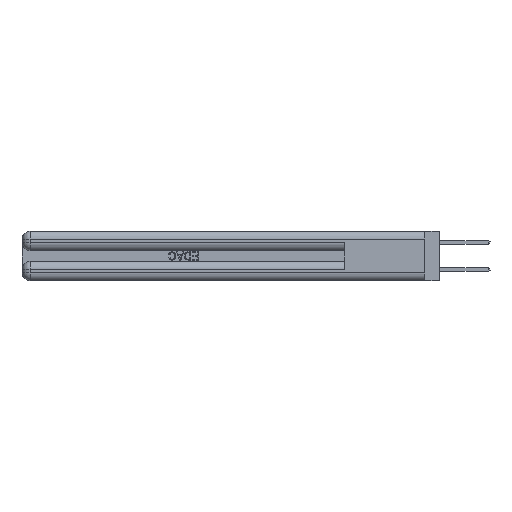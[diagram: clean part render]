
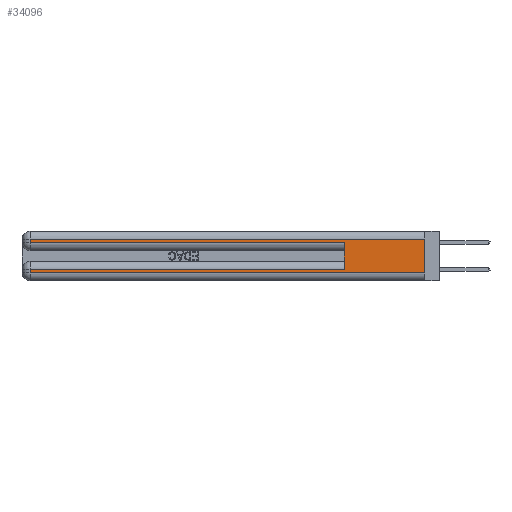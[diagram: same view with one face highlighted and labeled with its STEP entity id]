
A CAD part, left-side view. The second image highlights one B-rep face of the part: STEP entity #34096.
In plain terms, the highlighted planar face has unit normal (-1, 0, 0).
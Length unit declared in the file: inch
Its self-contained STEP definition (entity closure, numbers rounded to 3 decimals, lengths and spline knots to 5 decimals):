
#402 = ORIENTED_EDGE ( 'NONE', *, *, #39180, .T. ) ;
#793 = VERTEX_POINT ( 'NONE', #20027 ) ;
#1007 = EDGE_CURVE ( 'NONE', #11120, #20701, #22849, .T. ) ;
#1410 = LINE ( 'NONE', #12347, #18980 ) ;
#1851 = DIRECTION ( 'NONE',  ( 0., -1., 0. ) ) ;
#2838 = LINE ( 'NONE', #35011, #39089 ) ;
#2894 = ORIENTED_EDGE ( 'NONE', *, *, #20124, .T. ) ;
#4474 = CARTESIAN_POINT ( 'NONE',  ( 0., 2.94, 0.285 ) ) ;
#4774 = EDGE_CURVE ( 'NONE', #20701, #21897, #1410, .T. ) ;
#4783 = ORIENTED_EDGE ( 'NONE', *, *, #1007, .T. ) ;
#5353 = CARTESIAN_POINT ( 'NONE',  ( 0., 0.6, 0.145 ) ) ;
#5579 = CARTESIAN_POINT ( 'NONE',  ( 0., 2.94, 0.37 ) ) ;
#5633 = VERTEX_POINT ( 'NONE', #28132 ) ;
#5831 = CARTESIAN_POINT ( 'NONE',  ( 0., 0.6, 0.285 ) ) ;
#7106 = ORIENTED_EDGE ( 'NONE', *, *, #4774, .T. ) ;
#7929 = DIRECTION ( 'NONE',  ( 1., 0., 0. ) ) ;
#8664 = DIRECTION ( 'NONE',  ( 0., 0., -1. ) ) ;
#9414 = VERTEX_POINT ( 'NONE', #5831 ) ;
#10093 = VERTEX_POINT ( 'NONE', #29046 ) ;
#10469 = LINE ( 'NONE', #5353, #12691 ) ;
#11120 = VERTEX_POINT ( 'NONE', #17565 ) ;
#12266 = DIRECTION ( 'NONE',  ( 0., 1., 0. ) ) ;
#12347 = CARTESIAN_POINT ( 'NONE',  ( 0., 2.94, 0.37 ) ) ;
#12691 = VECTOR ( 'NONE', #19788, 39.37008 ) ;
#13507 = VECTOR ( 'NONE', #12266, 39.37008 ) ;
#14107 = EDGE_CURVE ( 'NONE', #10093, #793, #14462, .T. ) ;
#14462 = LINE ( 'NONE', #36508, #32043 ) ;
#17565 = CARTESIAN_POINT ( 'NONE',  ( 0., 0.6, 0.085 ) ) ;
#18980 = VECTOR ( 'NONE', #8664, 39.37008 ) ;
#19788 = DIRECTION ( 'NONE',  ( 0., 0., 1. ) ) ;
#19977 = EDGE_CURVE ( 'NONE', #793, #39813, #20931, .T. ) ;
#20027 = CARTESIAN_POINT ( 'NONE',  ( 0., 2.94, 0.31 ) ) ;
#20124 = EDGE_CURVE ( 'NONE', #21897, #5633, #37459, .T. ) ;
#20701 = VERTEX_POINT ( 'NONE', #36445 ) ;
#20931 = LINE ( 'NONE', #5579, #44081 ) ;
#21469 = PLANE ( 'NONE',  #40001 ) ;
#21581 = CARTESIAN_POINT ( 'NONE',  ( 0., 0., 0.285 ) ) ;
#21897 = VERTEX_POINT ( 'NONE', #40116 ) ;
#22849 = LINE ( 'NONE', #29802, #13507 ) ;
#23555 = DIRECTION ( 'NONE',  ( 0., 0., -1. ) ) ;
#23606 = ORIENTED_EDGE ( 'NONE', *, *, #19977, .T. ) ;
#25452 = DIRECTION ( 'NONE',  ( 0., 0., -1. ) ) ;
#28089 = DIRECTION ( 'NONE',  ( 0., 0., -1. ) ) ;
#28132 = CARTESIAN_POINT ( 'NONE',  ( 0., 0., 0.06 ) ) ;
#29046 = CARTESIAN_POINT ( 'NONE',  ( 0., 0., 0.31 ) ) ;
#29332 = FACE_OUTER_BOUND ( 'NONE', #40076, .T. ) ;
#29719 = EDGE_CURVE ( 'NONE', #10093, #5633, #2838, .T. ) ;
#29745 = DIRECTION ( 'NONE',  ( 0., -1., 0. ) ) ;
#29802 = CARTESIAN_POINT ( 'NONE',  ( 0., 0., 0.085 ) ) ;
#32043 = VECTOR ( 'NONE', #40526, 39.37008 ) ;
#34096 = ADVANCED_FACE ( 'NONE', ( #29332 ), #21469, .F. ) ;
#35011 = CARTESIAN_POINT ( 'NONE',  ( 0., 0., 0.37 ) ) ;
#36310 = VECTOR ( 'NONE', #1851, 39.37008 ) ;
#36445 = CARTESIAN_POINT ( 'NONE',  ( 0., 2.94, 0.085 ) ) ;
#36508 = CARTESIAN_POINT ( 'NONE',  ( 0., 0., 0.31 ) ) ;
#37459 = LINE ( 'NONE', #43812, #36310 ) ;
#38442 = ORIENTED_EDGE ( 'NONE', *, *, #44575, .F. ) ;
#39089 = VECTOR ( 'NONE', #28089, 39.37008 ) ;
#39156 = CARTESIAN_POINT ( 'NONE',  ( 0., 0., 0.37 ) ) ;
#39180 = EDGE_CURVE ( 'NONE', #39813, #9414, #41886, .T. ) ;
#39452 = ORIENTED_EDGE ( 'NONE', *, *, #29719, .F. ) ;
#39813 = VERTEX_POINT ( 'NONE', #4474 ) ;
#40001 = AXIS2_PLACEMENT_3D ( 'NONE', #39156, #7929, #25452 ) ;
#40076 = EDGE_LOOP ( 'NONE', ( #39452, #40682, #23606, #402, #38442, #4783, #7106, #2894 ) ) ;
#40116 = CARTESIAN_POINT ( 'NONE',  ( 0., 2.94, 0.06 ) ) ;
#40526 = DIRECTION ( 'NONE',  ( 0., 1., 0. ) ) ;
#40682 = ORIENTED_EDGE ( 'NONE', *, *, #14107, .T. ) ;
#40802 = VECTOR ( 'NONE', #29745, 39.37008 ) ;
#41886 = LINE ( 'NONE', #21581, #40802 ) ;
#43812 = CARTESIAN_POINT ( 'NONE',  ( 0., 0., 0.06 ) ) ;
#44081 = VECTOR ( 'NONE', #23555, 39.37008 ) ;
#44575 = EDGE_CURVE ( 'NONE', #11120, #9414, #10469, .T. ) ;
